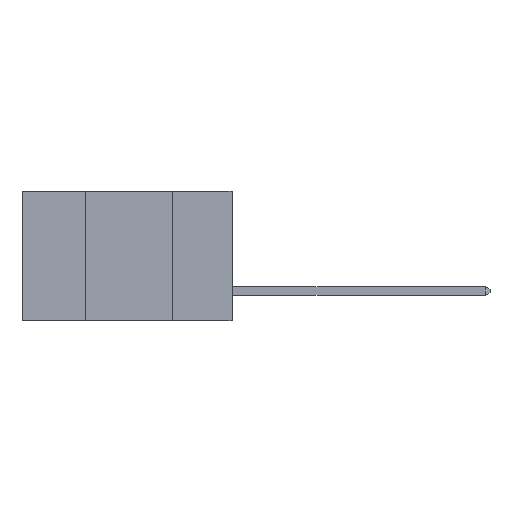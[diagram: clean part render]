
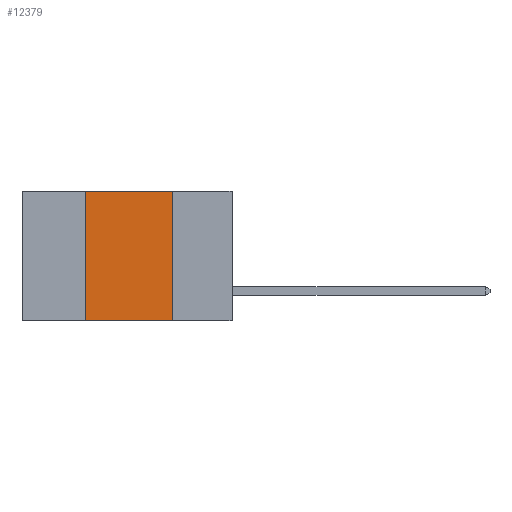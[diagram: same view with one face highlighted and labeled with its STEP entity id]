
A CAD part, left-side view. The second image highlights one B-rep face of the part: STEP entity #12379.
In plain terms, the highlighted planar face has unit normal (-1, 0, 0).
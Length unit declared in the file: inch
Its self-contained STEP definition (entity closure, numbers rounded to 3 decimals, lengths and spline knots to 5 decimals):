
#73 = VERTEX_POINT ( 'NONE', #2508 ) ;
#421 = CARTESIAN_POINT ( 'NONE',  ( 0., 0.42, -0.37 ) ) ;
#907 = CARTESIAN_POINT ( 'NONE',  ( 0., 0.42, 0. ) ) ;
#931 = FACE_OUTER_BOUND ( 'NONE', #11229, .T. ) ;
#2508 = CARTESIAN_POINT ( 'NONE',  ( 0., 0.17, -0.37 ) ) ;
#3544 = VERTEX_POINT ( 'NONE', #4201 ) ;
#3660 = LINE ( 'NONE', #13047, #6366 ) ;
#4022 = AXIS2_PLACEMENT_3D ( 'NONE', #4165, #11273, #5209 ) ;
#4165 = CARTESIAN_POINT ( 'NONE',  ( 0., 0.6, 0. ) ) ;
#4201 = CARTESIAN_POINT ( 'NONE',  ( 0., 0.17, 0. ) ) ;
#4500 = VERTEX_POINT ( 'NONE', #421 ) ;
#4945 = VECTOR ( 'NONE', #11232, 39.37008 ) ;
#5209 = DIRECTION ( 'NONE',  ( 0., 0., -1. ) ) ;
#5214 = EDGE_CURVE ( 'NONE', #3544, #73, #6527, .T. ) ;
#5313 = EDGE_CURVE ( 'NONE', #4500, #7731, #12912, .T. ) ;
#5890 = VECTOR ( 'NONE', #8459, 39.37008 ) ;
#6068 = DIRECTION ( 'NONE',  ( 0., -1., 0. ) ) ;
#6366 = VECTOR ( 'NONE', #6068, 39.37008 ) ;
#6527 = LINE ( 'NONE', #11816, #5890 ) ;
#7062 = EDGE_CURVE ( 'NONE', #4500, #73, #7329, .T. ) ;
#7329 = LINE ( 'NONE', #11211, #9696 ) ;
#7731 = VERTEX_POINT ( 'NONE', #907 ) ;
#8082 = ORIENTED_EDGE ( 'NONE', *, *, #9831, .F. ) ;
#8459 = DIRECTION ( 'NONE',  ( 0., 0., -1. ) ) ;
#8719 = ORIENTED_EDGE ( 'NONE', *, *, #7062, .T. ) ;
#9696 = VECTOR ( 'NONE', #13143, 39.37008 ) ;
#9831 = EDGE_CURVE ( 'NONE', #7731, #3544, #3660, .T. ) ;
#10294 = PLANE ( 'NONE',  #4022 ) ;
#10755 = ORIENTED_EDGE ( 'NONE', *, *, #5313, .F. ) ;
#11211 = CARTESIAN_POINT ( 'NONE',  ( 0., 0.6, -0.37 ) ) ;
#11229 = EDGE_LOOP ( 'NONE', ( #12992, #8082, #10755, #8719 ) ) ;
#11232 = DIRECTION ( 'NONE',  ( 0., 0., 1. ) ) ;
#11273 = DIRECTION ( 'NONE',  ( 1., 0., 0. ) ) ;
#11816 = CARTESIAN_POINT ( 'NONE',  ( 0., 0.17, 0. ) ) ;
#12027 = CARTESIAN_POINT ( 'NONE',  ( 0., 0.42, 0. ) ) ;
#12379 = ADVANCED_FACE ( 'NONE', ( #931 ), #10294, .F. ) ;
#12912 = LINE ( 'NONE', #12027, #4945 ) ;
#12992 = ORIENTED_EDGE ( 'NONE', *, *, #5214, .F. ) ;
#13047 = CARTESIAN_POINT ( 'NONE',  ( 0., 0.6, 0. ) ) ;
#13143 = DIRECTION ( 'NONE',  ( 0., -1., 0. ) ) ;
